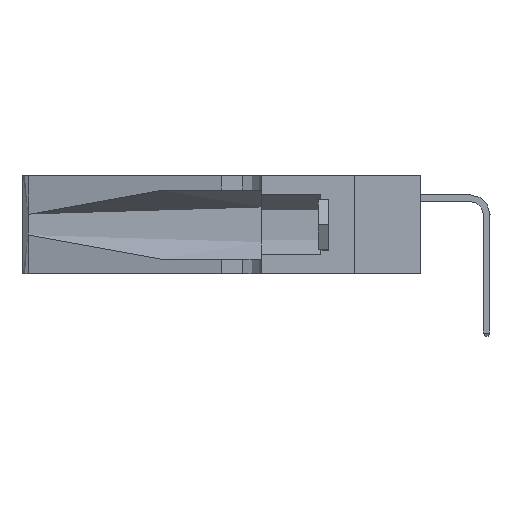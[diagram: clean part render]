
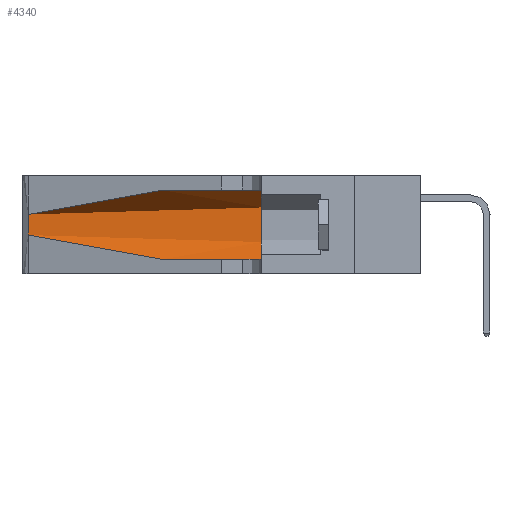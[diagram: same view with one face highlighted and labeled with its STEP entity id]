
A CAD part, left-side view. The second image highlights one B-rep face of the part: STEP entity #4340.
In plain terms, the highlighted cylindrical face has radius 3.308 mm (diameter 6.617 mm), a partial arc.
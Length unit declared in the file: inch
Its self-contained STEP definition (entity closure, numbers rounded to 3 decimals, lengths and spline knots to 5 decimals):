
#126 = CARTESIAN_POINT ( 'NONE',  ( 0.25487, 1.22718, 0.22369 ) ) ;
#542 = VECTOR ( 'NONE', #6276, 39.37008 ) ;
#1182 = CARTESIAN_POINT ( 'NONE',  ( 0.25487, 1.22718, 0.22369 ) ) ;
#1943 = CARTESIAN_POINT ( 'NONE',  ( 0.26075, 1.23896, 0.178 ) ) ;
#3053 = ORIENTED_EDGE ( 'NONE', *, *, #11792, .T. ) ;
#3188 = CARTESIAN_POINT ( 'NONE',  ( 0.1305, 1.61858, 0.31525 ) ) ;
#4340 = ADVANCED_FACE ( 'NONE', ( #28458 ), #27551, .F. ) ;
#5027 = CARTESIAN_POINT ( 'NONE',  ( 0.25856, 1.23593, 0.16098 ) ) ;
#6276 = DIRECTION ( 'NONE',  ( 0., -1., 0. ) ) ;
#6580 = ORIENTED_EDGE ( 'NONE', *, *, #31337, .T. ) ;
#7179 = CARTESIAN_POINT ( 'NONE',  ( 0.1305, 0.72297, 0.31525 ) ) ;
#8115 = CARTESIAN_POINT ( 'NONE',  ( 0.25639, 1.23186, 0.15144 ) ) ;
#8248 = VERTEX_POINT ( 'NONE', #36360 ) ;
#8362 = ORIENTED_EDGE ( 'NONE', *, *, #31288, .T. ) ;
#9910 = EDGE_LOOP ( 'NONE', ( #12285, #3053, #8362, #6580, #20642, #25773 ) ) ;
#10102 = B_SPLINE_CURVE_WITH_KNOTS ( 'NONE', 3,
 ( #13993, #28564, #13867, #34397, #17005, #37276, #19967, #1943, #22884, #5027, #25785, #8115, #28682, #11147 ),
 .UNSPECIFIED., .F., .F.,
 ( 4, 2, 2, 2, 2, 2, 4 ),
 ( 0., 0.00027, 0.00053, 0.00107, 0.0016, 0.00187, 0.00214 ),
 .UNSPECIFIED. ) ;
#10127 = DIRECTION ( 'NONE',  ( 0., -1., 0. ) ) ;
#11147 = CARTESIAN_POINT ( 'NONE',  ( 0.25487, 1.22718, 0.14631 ) ) ;
#11792 = EDGE_CURVE ( 'NONE', #22407, #15859, #10102, .T. ) ;
#11864 = CARTESIAN_POINT ( 'NONE',  ( 0.1305, 0.72297, 0.05475 ) ) ;
#12285 = ORIENTED_EDGE ( 'NONE', *, *, #31568, .T. ) ;
#12590 = CIRCLE ( 'NONE', #33599, 0.13025 ) ;
#13867 = CARTESIAN_POINT ( 'NONE',  ( 0.25639, 1.23184, 0.21858 ) ) ;
#13993 = CARTESIAN_POINT ( 'NONE',  ( 0.25487, 1.22718, 0.22369 ) ) ;
#15782 = AXIS2_PLACEMENT_3D ( 'NONE', #17177, #37440, #20141 ) ;
#15859 = VERTEX_POINT ( 'NONE', #20072 ) ;
#16625 = LINE ( 'NONE', #3188, #542 ) ;
#17005 = CARTESIAN_POINT ( 'NONE',  ( 0.25854, 1.2359, 0.20912 ) ) ;
#17035 = CARTESIAN_POINT ( 'NONE',  ( 0.1305, 0.35, 0.185 ) ) ;
#17177 = CARTESIAN_POINT ( 'NONE',  ( 0.1305, 1.61858, 0.185 ) ) ;
#17708 = CARTESIAN_POINT ( 'NONE',  ( 0.25487, 1.22718, 0.14631 ) ) ;
#19212 = CARTESIAN_POINT ( 'NONE',  ( 0.2373, 1.15595, 0.28018 ) ) ;
#19510 = VECTOR ( 'NONE', #10127, 39.37008 ) ;
#19613 = CARTESIAN_POINT ( 'NONE',  ( 0.1305, 0.72297, 0.31525 ) ) ;
#19967 = CARTESIAN_POINT ( 'NONE',  ( 0.26075, 1.23896, 0.19203 ) ) ;
#19996 = DIRECTION ( 'NONE',  ( 0., 0., 1. ) ) ;
#20072 = CARTESIAN_POINT ( 'NONE',  ( 0.25487, 1.22718, 0.14631 ) ) ;
#20141 = DIRECTION ( 'NONE',  ( 0., 0., -1. ) ) ;
#20642 = ORIENTED_EDGE ( 'NONE', *, *, #30886, .F. ) ;
#22407 = VERTEX_POINT ( 'NONE', #126 ) ;
#22884 = CARTESIAN_POINT ( 'NONE',  ( 0.26017, 1.23833, 0.17102 ) ) ;
#25773 = ORIENTED_EDGE ( 'NONE', *, *, #36560, .F. ) ;
#25785 = CARTESIAN_POINT ( 'NONE',  ( 0.25789, 1.23486, 0.15765 ) ) ;
#26317 = CARTESIAN_POINT ( 'NONE',  ( 0.1305, 0.35, 0.05475 ) ) ;
#26437 = VERTEX_POINT ( 'NONE', #30877 ) ;
#26467 = CARTESIAN_POINT ( 'NONE',  ( 0.2373, 1.15595, 0.08982 ) ) ;
#27152 =( BOUNDED_CURVE ( )  B_SPLINE_CURVE ( 3, ( #17708, #26467, #29380, #11864 ),
 .UNSPECIFIED., .F., .T. ) 
 B_SPLINE_CURVE_WITH_KNOTS ( ( 4, 4 ),
 ( 3.44316, 4.71239 ),
 .UNSPECIFIED. ) 
 CURVE ( )  GEOMETRIC_REPRESENTATION_ITEM ( )  RATIONAL_B_SPLINE_CURVE ( ( 1., 0.87, 0.87, 1. ) ) 
 REPRESENTATION_ITEM ( '' )  );
#27213 = LINE ( 'NONE', #29512, #19510 ) ;
#27252 =( BOUNDED_CURVE ( )  B_SPLINE_CURVE ( 3, ( #7179, #36412, #19212, #1182 ),
 .UNSPECIFIED., .F., .T. ) 
 B_SPLINE_CURVE_WITH_KNOTS ( ( 4, 4 ),
 ( 1.5708, 2.84003 ),
 .UNSPECIFIED. ) 
 CURVE ( )  GEOMETRIC_REPRESENTATION_ITEM ( )  RATIONAL_B_SPLINE_CURVE ( ( 1., 0.87, 0.87, 1. ) ) 
 REPRESENTATION_ITEM ( '' )  );
#27551 = CYLINDRICAL_SURFACE ( 'NONE', #15782, 0.13025 ) ;
#28458 = FACE_OUTER_BOUND ( 'NONE', #9910, .T. ) ;
#28564 = CARTESIAN_POINT ( 'NONE',  ( 0.25555, 1.22994, 0.2215 ) ) ;
#28682 = CARTESIAN_POINT ( 'NONE',  ( 0.25555, 1.22993, 0.14849 ) ) ;
#29087 = VERTEX_POINT ( 'NONE', #26317 ) ;
#29380 = CARTESIAN_POINT ( 'NONE',  ( 0.18966, 0.96281, 0.05475 ) ) ;
#29512 = CARTESIAN_POINT ( 'NONE',  ( 0.1305, 1.61858, 0.05475 ) ) ;
#30877 = CARTESIAN_POINT ( 'NONE',  ( 0.1305, 0.35, 0.31525 ) ) ;
#30886 = EDGE_CURVE ( 'NONE', #26437, #29087, #12590, .T. ) ;
#31288 = EDGE_CURVE ( 'NONE', #15859, #8248, #27152, .T. ) ;
#31337 = EDGE_CURVE ( 'NONE', #8248, #29087, #27213, .T. ) ;
#31568 = EDGE_CURVE ( 'NONE', #38279, #22407, #27252, .T. ) ;
#33599 = AXIS2_PLACEMENT_3D ( 'NONE', #17035, #37303, #19996 ) ;
#34397 = CARTESIAN_POINT ( 'NONE',  ( 0.25787, 1.23484, 0.2124 ) ) ;
#36360 = CARTESIAN_POINT ( 'NONE',  ( 0.1305, 0.72297, 0.05475 ) ) ;
#36412 = CARTESIAN_POINT ( 'NONE',  ( 0.18966, 0.96281, 0.31525 ) ) ;
#36560 = EDGE_CURVE ( 'NONE', #38279, #26437, #16625, .T. ) ;
#37276 = CARTESIAN_POINT ( 'NONE',  ( 0.26018, 1.23835, 0.19895 ) ) ;
#37303 = DIRECTION ( 'NONE',  ( 0., 1., 0. ) ) ;
#37440 = DIRECTION ( 'NONE',  ( 0., -1., 0. ) ) ;
#38279 = VERTEX_POINT ( 'NONE', #19613 ) ;
